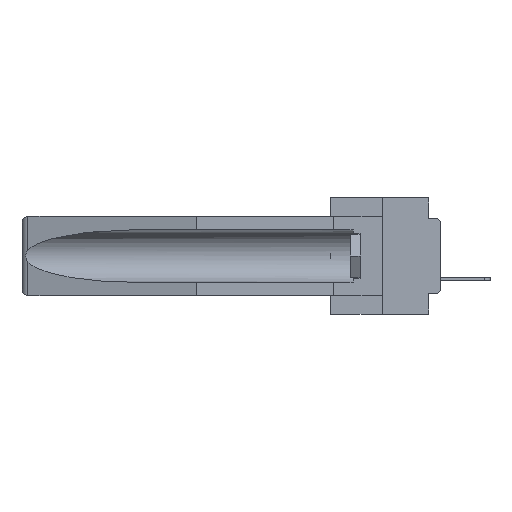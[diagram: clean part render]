
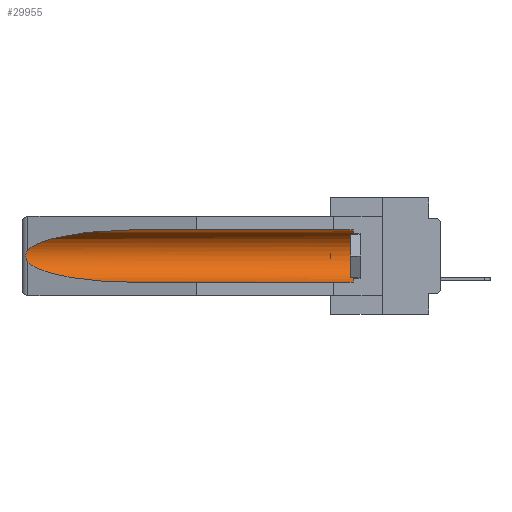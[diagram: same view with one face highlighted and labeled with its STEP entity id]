
A CAD part, left-side view. The second image highlights one B-rep face of the part: STEP entity #29955.
In plain terms, the highlighted cylindrical face has radius 2.857 mm (diameter 5.715 mm), a partial arc.
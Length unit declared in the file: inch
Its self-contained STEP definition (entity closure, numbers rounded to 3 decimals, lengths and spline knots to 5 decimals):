
#168 = CARTESIAN_POINT ( 'NONE',  ( 0.2673, 1.53269, -0.17917 ) ) ;
#308 = EDGE_CURVE ( 'NONE', #28130, #29242, #5141, .T. ) ;
#1003 = CARTESIAN_POINT ( 'NONE',  ( 0.155, 1.07973, -0.284 ) ) ;
#1365 = CARTESIAN_POINT ( 'NONE',  ( 0.155, -0.30754, -0.1715 ) ) ;
#1694 = CARTESIAN_POINT ( 'NONE',  ( 0.21114, 1.30732, -0.059 ) ) ;
#1932 =( BOUNDED_CURVE ( )  B_SPLINE_CURVE ( 3, ( #19991, #1694, #38585, #29775 ),
 .UNSPECIFIED., .F., .F. ) 
 B_SPLINE_CURVE_WITH_KNOTS ( ( 4, 4 ),
 ( 4.71239, 6.08839 ),
 .UNSPECIFIED. ) 
 CURVE ( )  GEOMETRIC_REPRESENTATION_ITEM ( )  RATIONAL_B_SPLINE_CURVE ( ( 1., 0.848, 0.848, 1. ) ) 
 REPRESENTATION_ITEM ( '' )  );
#3123 = CARTESIAN_POINT ( 'NONE',  ( 0.26597, 1.52961, -0.15275 ) ) ;
#3264 = CARTESIAN_POINT ( 'NONE',  ( 0.26597, 1.5296, -0.19026 ) ) ;
#3448 = EDGE_CURVE ( 'NONE', #7917, #29242, #36469, .T. ) ;
#5141 = LINE ( 'NONE', #30856, #14734 ) ;
#5710 = CARTESIAN_POINT ( 'NONE',  ( 0.155, 0.126, -0.284 ) ) ;
#5841 = DIRECTION ( 'NONE',  ( 0., 1., 0. ) ) ;
#6358 = VERTEX_POINT ( 'NONE', #6466 ) ;
#6466 = CARTESIAN_POINT ( 'NONE',  ( 0.155, 0.126, -0.059 ) ) ;
#6888 = EDGE_LOOP ( 'NONE', ( #9702, #12134, #30525, #31329, #14329, #36468 ) ) ;
#6964 = VECTOR ( 'NONE', #35689, 39.37008 ) ;
#7412 = CARTESIAN_POINT ( 'NONE',  ( 0.155, 1.07973, -0.284 ) ) ;
#7917 = VERTEX_POINT ( 'NONE', #39472 ) ;
#8845 = EDGE_CURVE ( 'NONE', #28130, #6358, #37920, .T. ) ;
#9324 = CARTESIAN_POINT ( 'NONE',  ( 0.2673, 1.5327, -0.16383 ) ) ;
#9702 = ORIENTED_EDGE ( 'NONE', *, *, #14521, .T. ) ;
#10411 = CARTESIAN_POINT ( 'NONE',  ( 0.25451, 1.48313, -0.24835 ) ) ;
#12044 = VERTEX_POINT ( 'NONE', #37720 ) ;
#12134 = ORIENTED_EDGE ( 'NONE', *, *, #14797, .T. ) ;
#14117 = DIRECTION ( 'NONE',  ( 0., -1., 0. ) ) ;
#14329 = ORIENTED_EDGE ( 'NONE', *, *, #8845, .T. ) ;
#14521 = EDGE_CURVE ( 'NONE', #12044, #32755, #1932, .T. ) ;
#14734 = VECTOR ( 'NONE', #5841, 39.37008 ) ;
#14797 = EDGE_CURVE ( 'NONE', #32755, #7917, #26345, .T. ) ;
#15483 = CARTESIAN_POINT ( 'NONE',  ( 0.2675, 1.53308, -0.17534 ) ) ;
#15622 = CARTESIAN_POINT ( 'NONE',  ( 0.26654, 1.53092, -0.15636 ) ) ;
#16944 = DIRECTION ( 'NONE',  ( 0., 0., 1. ) ) ;
#18452 = CARTESIAN_POINT ( 'NONE',  ( 0.26537, 1.52718, -0.14972 ) ) ;
#18735 = CARTESIAN_POINT ( 'NONE',  ( 0.26537, 1.52718, -0.19328 ) ) ;
#19991 = CARTESIAN_POINT ( 'NONE',  ( 0.155, 1.07973, -0.059 ) ) ;
#20312 = CARTESIAN_POINT ( 'NONE',  ( 0.155, 0.126, -0.1715 ) ) ;
#21664 = CARTESIAN_POINT ( 'NONE',  ( 0.26655, 1.53094, -0.18657 ) ) ;
#22892 = CARTESIAN_POINT ( 'NONE',  ( 0.21114, 1.30732, -0.284 ) ) ;
#23043 = CARTESIAN_POINT ( 'NONE',  ( 0.155, -0.30754, -0.059 ) ) ;
#24281 = CYLINDRICAL_SURFACE ( 'NONE', #39825, 0.1125 ) ;
#24460 = AXIS2_PLACEMENT_3D ( 'NONE', #20312, #14117, #38655 ) ;
#26345 = B_SPLINE_CURVE_WITH_KNOTS ( 'NONE', 3,
 ( #18452, #3123, #15622, #9324, #30816, #15483, #168, #21664, #3264, #18735 ),
 .UNSPECIFIED., .F., .F.,
 ( 4, 2, 2, 2, 4 ),
 ( 0., 0.00029, 0.00058, 0.00087, 0.00117 ),
 .UNSPECIFIED. ) ;
#28130 = VERTEX_POINT ( 'NONE', #5710 ) ;
#29151 = CARTESIAN_POINT ( 'NONE',  ( 0.26537, 1.52718, -0.14972 ) ) ;
#29242 = VERTEX_POINT ( 'NONE', #1003 ) ;
#29446 = DIRECTION ( 'NONE',  ( 0., 1., 0. ) ) ;
#29593 = LINE ( 'NONE', #23043, #6964 ) ;
#29775 = CARTESIAN_POINT ( 'NONE',  ( 0.26537, 1.52718, -0.14972 ) ) ;
#29955 = ADVANCED_FACE ( 'NONE', ( #31990 ), #24281, .F. ) ;
#30525 = ORIENTED_EDGE ( 'NONE', *, *, #3448, .T. ) ;
#30816 = CARTESIAN_POINT ( 'NONE',  ( 0.2675, 1.53308, -0.16763 ) ) ;
#30856 = CARTESIAN_POINT ( 'NONE',  ( 0.155, -0.30754, -0.284 ) ) ;
#31329 = ORIENTED_EDGE ( 'NONE', *, *, #308, .F. ) ;
#31990 = FACE_OUTER_BOUND ( 'NONE', #6888, .T. ) ;
#32755 = VERTEX_POINT ( 'NONE', #29151 ) ;
#35689 = DIRECTION ( 'NONE',  ( 0., 1., 0. ) ) ;
#36468 = ORIENTED_EDGE ( 'NONE', *, *, #37534, .T. ) ;
#36469 =( BOUNDED_CURVE ( )  B_SPLINE_CURVE ( 3, ( #37854, #10411, #22892, #7412 ),
 .UNSPECIFIED., .F., .F. ) 
 B_SPLINE_CURVE_WITH_KNOTS ( ( 4, 4 ),
 ( 0.1948, 1.5708 ),
 .UNSPECIFIED. ) 
 CURVE ( )  GEOMETRIC_REPRESENTATION_ITEM ( )  RATIONAL_B_SPLINE_CURVE ( ( 1., 0.848, 0.848, 1. ) ) 
 REPRESENTATION_ITEM ( '' )  );
#37534 = EDGE_CURVE ( 'NONE', #6358, #12044, #29593, .T. ) ;
#37720 = CARTESIAN_POINT ( 'NONE',  ( 0.155, 1.07973, -0.059 ) ) ;
#37854 = CARTESIAN_POINT ( 'NONE',  ( 0.26537, 1.52718, -0.19328 ) ) ;
#37920 = CIRCLE ( 'NONE', #24460, 0.1125 ) ;
#38585 = CARTESIAN_POINT ( 'NONE',  ( 0.25451, 1.48313, -0.09465 ) ) ;
#38655 = DIRECTION ( 'NONE',  ( 0., 0., 1. ) ) ;
#39472 = CARTESIAN_POINT ( 'NONE',  ( 0.26537, 1.52718, -0.19328 ) ) ;
#39825 = AXIS2_PLACEMENT_3D ( 'NONE', #1365, #29446, #16944 ) ;
